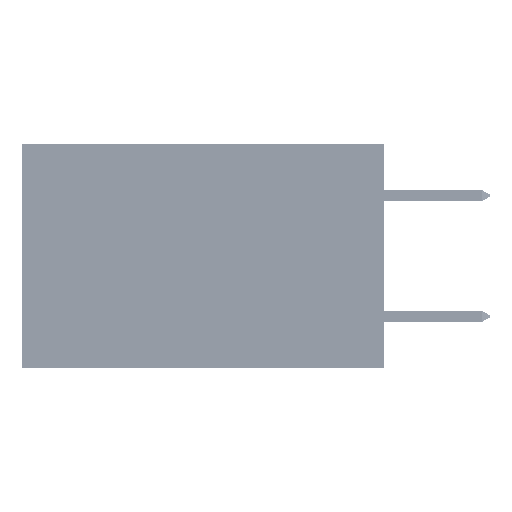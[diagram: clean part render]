
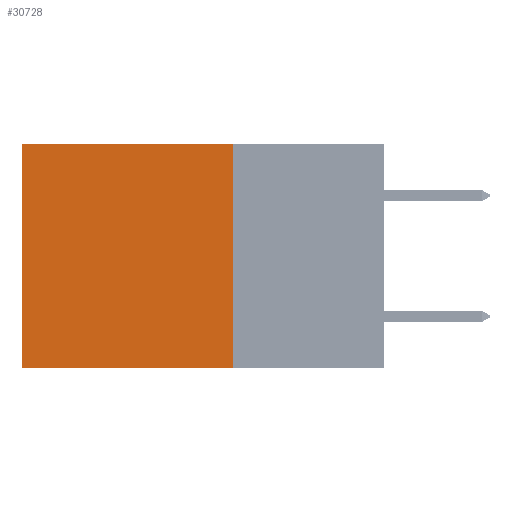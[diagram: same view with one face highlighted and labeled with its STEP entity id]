
A CAD part, left-side view. The second image highlights one B-rep face of the part: STEP entity #30728.
In plain terms, the highlighted planar face has unit normal (-1, 0, 0).
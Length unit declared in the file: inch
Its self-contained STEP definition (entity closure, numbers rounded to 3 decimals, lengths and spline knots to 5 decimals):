
#74 = VECTOR ( 'NONE', #13204, 39.37008 ) ;
#1607 = ORIENTED_EDGE ( 'NONE', *, *, #37085, .T. ) ;
#2715 = CARTESIAN_POINT ( 'NONE',  ( 0.2875, 0.6, -0.37 ) ) ;
#3790 = ORIENTED_EDGE ( 'NONE', *, *, #46509, .F. ) ;
#5018 = VERTEX_POINT ( 'NONE', #15693 ) ;
#5641 = PLANE ( 'NONE',  #8435 ) ;
#6430 = LINE ( 'NONE', #10600, #24464 ) ;
#7320 = VECTOR ( 'NONE', #24027, 39.37008 ) ;
#8435 = AXIS2_PLACEMENT_3D ( 'NONE', #9534, #13396, #39949 ) ;
#9355 = CARTESIAN_POINT ( 'NONE',  ( 0.2875, 0.25, -0.37 ) ) ;
#9534 = CARTESIAN_POINT ( 'NONE',  ( 0.2875, 0.25, 0. ) ) ;
#10600 = CARTESIAN_POINT ( 'NONE',  ( 0.2875, 0.25, 0. ) ) ;
#13121 = FACE_OUTER_BOUND ( 'NONE', #41880, .T. ) ;
#13204 = DIRECTION ( 'NONE',  ( 0., 1., 0. ) ) ;
#13396 = DIRECTION ( 'NONE',  ( 1., 0., 0. ) ) ;
#15693 = CARTESIAN_POINT ( 'NONE',  ( 0.2875, 0.25, -0.37 ) ) ;
#16811 = VERTEX_POINT ( 'NONE', #40449 ) ;
#16934 = DIRECTION ( 'NONE',  ( 0., 0., -1. ) ) ;
#20194 = CARTESIAN_POINT ( 'NONE',  ( 0.2875, 0.25, 0. ) ) ;
#21841 = LINE ( 'NONE', #43367, #40722 ) ;
#22018 = DIRECTION ( 'NONE',  ( 0., 1., 0. ) ) ;
#23099 = ORIENTED_EDGE ( 'NONE', *, *, #40465, .T. ) ;
#24027 = DIRECTION ( 'NONE',  ( 0., 0., -1. ) ) ;
#24464 = VECTOR ( 'NONE', #22018, 39.37008 ) ;
#26283 = EDGE_CURVE ( 'NONE', #5018, #42481, #30788, .T. ) ;
#30728 = ADVANCED_FACE ( 'NONE', ( #13121 ), #5641, .F. ) ;
#30788 = LINE ( 'NONE', #9355, #74 ) ;
#32507 = CARTESIAN_POINT ( 'NONE',  ( 0.2875, 0.25, 0. ) ) ;
#37085 = EDGE_CURVE ( 'NONE', #16811, #42481, #21841, .T. ) ;
#39949 = DIRECTION ( 'NONE',  ( 0., 0., -1. ) ) ;
#40449 = CARTESIAN_POINT ( 'NONE',  ( 0.2875, 0.6, 0. ) ) ;
#40465 = EDGE_CURVE ( 'NONE', #46043, #16811, #6430, .T. ) ;
#40722 = VECTOR ( 'NONE', #16934, 39.37008 ) ;
#41880 = EDGE_LOOP ( 'NONE', ( #1607, #48128, #3790, #23099 ) ) ;
#42481 = VERTEX_POINT ( 'NONE', #2715 ) ;
#43367 = CARTESIAN_POINT ( 'NONE',  ( 0.2875, 0.6, 0. ) ) ;
#46043 = VERTEX_POINT ( 'NONE', #32507 ) ;
#46433 = LINE ( 'NONE', #20194, #7320 ) ;
#46509 = EDGE_CURVE ( 'NONE', #46043, #5018, #46433, .T. ) ;
#48128 = ORIENTED_EDGE ( 'NONE', *, *, #26283, .F. ) ;
